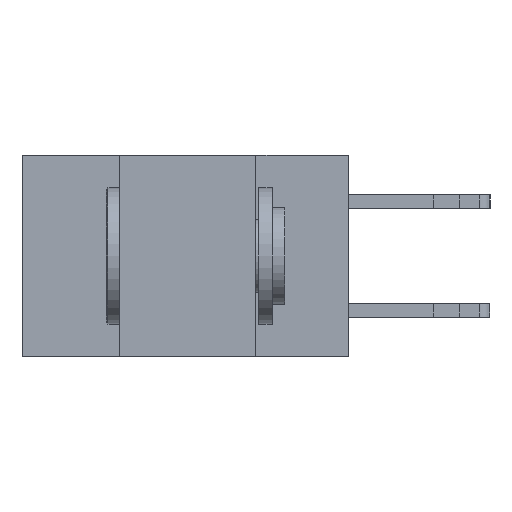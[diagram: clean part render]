
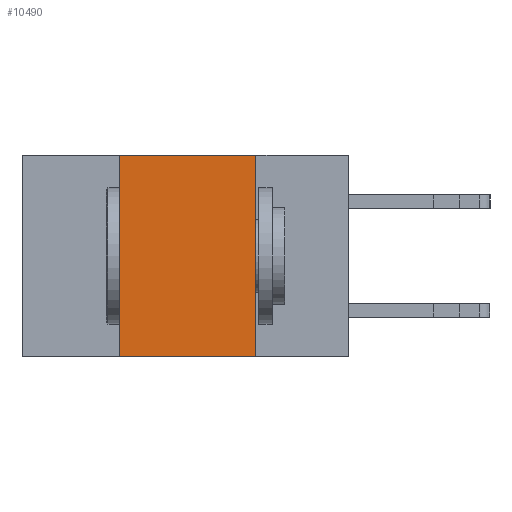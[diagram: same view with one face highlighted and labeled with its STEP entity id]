
A CAD part, left-side view. The second image highlights one B-rep face of the part: STEP entity #10490.
In plain terms, the highlighted planar face has unit normal (-1, 0, 0).
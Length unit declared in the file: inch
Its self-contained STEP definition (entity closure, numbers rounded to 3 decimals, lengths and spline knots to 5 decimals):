
#769 = CARTESIAN_POINT ( 'NONE',  ( 0., 0.17, -0.37 ) ) ;
#1073 = CARTESIAN_POINT ( 'NONE',  ( 0., 0.42, 0. ) ) ;
#1477 = EDGE_CURVE ( 'NONE', #17731, #8570, #10489, .T. ) ;
#1629 = AXIS2_PLACEMENT_3D ( 'NONE', #25893, #1735, #16059 ) ;
#1735 = DIRECTION ( 'NONE',  ( 1., 0., 0. ) ) ;
#4112 = DIRECTION ( 'NONE',  ( 0., 0., 1. ) ) ;
#4466 = VERTEX_POINT ( 'NONE', #8396 ) ;
#4917 = VECTOR ( 'NONE', #22684, 39.37008 ) ;
#6633 = DIRECTION ( 'NONE',  ( 0., -1., 0. ) ) ;
#6764 = CARTESIAN_POINT ( 'NONE',  ( 0., 0.6, 0. ) ) ;
#8396 = CARTESIAN_POINT ( 'NONE',  ( 0., 0.42, -0.37 ) ) ;
#8570 = VERTEX_POINT ( 'NONE', #769 ) ;
#8774 = CARTESIAN_POINT ( 'NONE',  ( 0., 0.6, -0.37 ) ) ;
#10489 = LINE ( 'NONE', #19877, #4917 ) ;
#10490 = ADVANCED_FACE ( 'NONE', ( #18279 ), #12050, .F. ) ;
#10685 = EDGE_CURVE ( 'NONE', #10834, #17731, #19815, .T. ) ;
#10834 = VERTEX_POINT ( 'NONE', #1073 ) ;
#10846 = ORIENTED_EDGE ( 'NONE', *, *, #14905, .T. ) ;
#11872 = EDGE_CURVE ( 'NONE', #4466, #10834, #22812, .T. ) ;
#12050 = PLANE ( 'NONE',  #1629 ) ;
#12303 = VECTOR ( 'NONE', #4112, 39.37008 ) ;
#14549 = VECTOR ( 'NONE', #18904, 39.37008 ) ;
#14905 = EDGE_CURVE ( 'NONE', #4466, #8570, #19929, .T. ) ;
#15904 = EDGE_LOOP ( 'NONE', ( #18666, #26070, #20823, #10846 ) ) ;
#16059 = DIRECTION ( 'NONE',  ( 0., 0., -1. ) ) ;
#17731 = VERTEX_POINT ( 'NONE', #19300 ) ;
#18279 = FACE_OUTER_BOUND ( 'NONE', #15904, .T. ) ;
#18666 = ORIENTED_EDGE ( 'NONE', *, *, #1477, .F. ) ;
#18904 = DIRECTION ( 'NONE',  ( 0., -1., 0. ) ) ;
#19300 = CARTESIAN_POINT ( 'NONE',  ( 0., 0.17, 0. ) ) ;
#19308 = VECTOR ( 'NONE', #6633, 39.37008 ) ;
#19815 = LINE ( 'NONE', #6764, #14549 ) ;
#19877 = CARTESIAN_POINT ( 'NONE',  ( 0., 0.17, 0. ) ) ;
#19929 = LINE ( 'NONE', #8774, #19308 ) ;
#20823 = ORIENTED_EDGE ( 'NONE', *, *, #11872, .F. ) ;
#22684 = DIRECTION ( 'NONE',  ( 0., 0., -1. ) ) ;
#22812 = LINE ( 'NONE', #26191, #12303 ) ;
#25893 = CARTESIAN_POINT ( 'NONE',  ( 0., 0.6, 0. ) ) ;
#26070 = ORIENTED_EDGE ( 'NONE', *, *, #10685, .F. ) ;
#26191 = CARTESIAN_POINT ( 'NONE',  ( 0., 0.42, 0. ) ) ;
